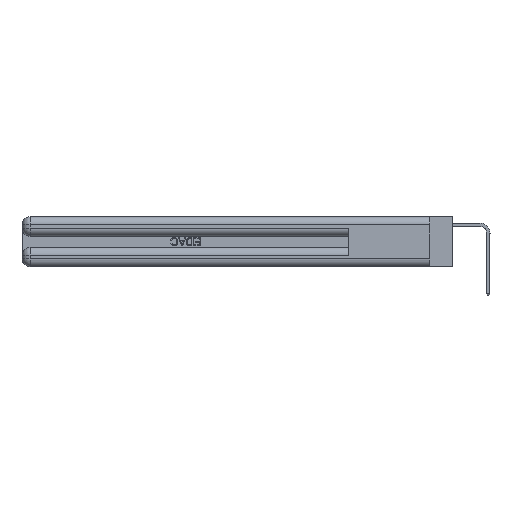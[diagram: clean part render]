
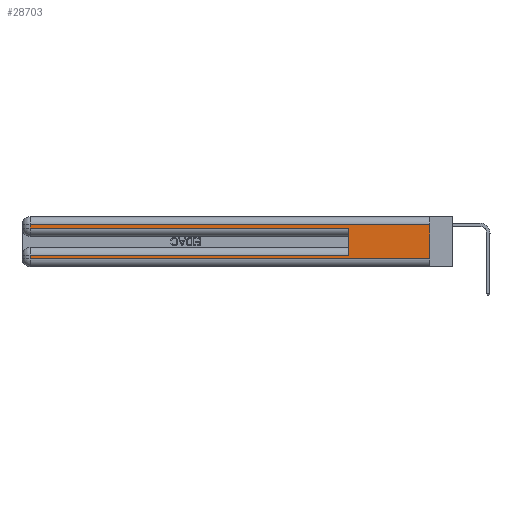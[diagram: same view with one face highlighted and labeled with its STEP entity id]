
A CAD part, left-side view. The second image highlights one B-rep face of the part: STEP entity #28703.
In plain terms, the highlighted planar face has unit normal (-1, 0, 0).
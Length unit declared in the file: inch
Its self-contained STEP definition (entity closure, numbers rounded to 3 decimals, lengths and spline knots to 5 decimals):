
#939 = CARTESIAN_POINT ( 'NONE',  ( 0., 2.94, 0.37 ) ) ;
#1863 = CARTESIAN_POINT ( 'NONE',  ( 0., 2.94, 0.285 ) ) ;
#2106 = VECTOR ( 'NONE', #22904, 39.37008 ) ;
#2240 = CARTESIAN_POINT ( 'NONE',  ( 0., 2.94, 0.31 ) ) ;
#2398 = DIRECTION ( 'NONE',  ( 0., 0., -1. ) ) ;
#3169 = VERTEX_POINT ( 'NONE', #1863 ) ;
#3526 = CARTESIAN_POINT ( 'NONE',  ( 0., 0.6, 0.085 ) ) ;
#4488 = EDGE_CURVE ( 'NONE', #3169, #23923, #26541, .T. ) ;
#4806 = VECTOR ( 'NONE', #12564, 39.37008 ) ;
#4996 = CARTESIAN_POINT ( 'NONE',  ( 0., 0., 0.06 ) ) ;
#5057 = CARTESIAN_POINT ( 'NONE',  ( 0., 0., 0.06 ) ) ;
#5118 = EDGE_CURVE ( 'NONE', #24408, #10112, #22521, .T. ) ;
#5964 = EDGE_CURVE ( 'NONE', #27807, #3169, #27616, .T. ) ;
#6028 = AXIS2_PLACEMENT_3D ( 'NONE', #30290, #17591, #2398 ) ;
#7339 = VECTOR ( 'NONE', #20966, 39.37008 ) ;
#7611 = LINE ( 'NONE', #10466, #20350 ) ;
#8115 = ORIENTED_EDGE ( 'NONE', *, *, #5118, .T. ) ;
#8141 = CARTESIAN_POINT ( 'NONE',  ( 0., 0., 0.31 ) ) ;
#9685 = VERTEX_POINT ( 'NONE', #8141 ) ;
#10076 = DIRECTION ( 'NONE',  ( 0., -1., 0. ) ) ;
#10112 = VERTEX_POINT ( 'NONE', #5057 ) ;
#10466 = CARTESIAN_POINT ( 'NONE',  ( 0., 0., 0.085 ) ) ;
#10651 = ORIENTED_EDGE ( 'NONE', *, *, #28915, .T. ) ;
#11354 = DIRECTION ( 'NONE',  ( 0., 1., 0. ) ) ;
#12394 = EDGE_LOOP ( 'NONE', ( #17187, #24290, #18702, #14174, #22247, #13338, #10651, #8115 ) ) ;
#12485 = PLANE ( 'NONE',  #6028 ) ;
#12564 = DIRECTION ( 'NONE',  ( 0., 0., -1. ) ) ;
#13027 = DIRECTION ( 'NONE',  ( 0., 1., 0. ) ) ;
#13338 = ORIENTED_EDGE ( 'NONE', *, *, #15269, .T. ) ;
#14124 = CARTESIAN_POINT ( 'NONE',  ( 0., 2.94, 0.085 ) ) ;
#14174 = ORIENTED_EDGE ( 'NONE', *, *, #4488, .T. ) ;
#15269 = EDGE_CURVE ( 'NONE', #24792, #23299, #7611, .T. ) ;
#17187 = ORIENTED_EDGE ( 'NONE', *, *, #21102, .F. ) ;
#17591 = DIRECTION ( 'NONE',  ( 1., 0., 0. ) ) ;
#18278 = LINE ( 'NONE', #27681, #4806 ) ;
#18402 = CARTESIAN_POINT ( 'NONE',  ( 0., 2.94, 0.37 ) ) ;
#18615 = LINE ( 'NONE', #939, #26958 ) ;
#18702 = ORIENTED_EDGE ( 'NONE', *, *, #5964, .T. ) ;
#20221 = CARTESIAN_POINT ( 'NONE',  ( 0., 0., 0.285 ) ) ;
#20350 = VECTOR ( 'NONE', #13027, 39.37008 ) ;
#20966 = DIRECTION ( 'NONE',  ( 0., 0., -1. ) ) ;
#21102 = EDGE_CURVE ( 'NONE', #9685, #10112, #18278, .T. ) ;
#21502 = CARTESIAN_POINT ( 'NONE',  ( 0., 0., 0.31 ) ) ;
#21755 = VECTOR ( 'NONE', #30412, 39.37008 ) ;
#22247 = ORIENTED_EDGE ( 'NONE', *, *, #25960, .F. ) ;
#22521 = LINE ( 'NONE', #4996, #21755 ) ;
#22853 = LINE ( 'NONE', #21502, #28807 ) ;
#22904 = DIRECTION ( 'NONE',  ( 0., 0., 1. ) ) ;
#23299 = VERTEX_POINT ( 'NONE', #14124 ) ;
#23923 = VERTEX_POINT ( 'NONE', #31677 ) ;
#23989 = LINE ( 'NONE', #25461, #2106 ) ;
#24212 = FACE_OUTER_BOUND ( 'NONE', #12394, .T. ) ;
#24290 = ORIENTED_EDGE ( 'NONE', *, *, #30891, .T. ) ;
#24408 = VERTEX_POINT ( 'NONE', #31744 ) ;
#24792 = VERTEX_POINT ( 'NONE', #3526 ) ;
#25461 = CARTESIAN_POINT ( 'NONE',  ( 0., 0.6, 0.145 ) ) ;
#25960 = EDGE_CURVE ( 'NONE', #24792, #23923, #23989, .T. ) ;
#26269 = DIRECTION ( 'NONE',  ( 0., 0., -1. ) ) ;
#26541 = LINE ( 'NONE', #20221, #32519 ) ;
#26958 = VECTOR ( 'NONE', #26269, 39.37008 ) ;
#27616 = LINE ( 'NONE', #18402, #7339 ) ;
#27681 = CARTESIAN_POINT ( 'NONE',  ( 0., 0., 0.37 ) ) ;
#27807 = VERTEX_POINT ( 'NONE', #2240 ) ;
#28703 = ADVANCED_FACE ( 'NONE', ( #24212 ), #12485, .F. ) ;
#28807 = VECTOR ( 'NONE', #11354, 39.37008 ) ;
#28915 = EDGE_CURVE ( 'NONE', #23299, #24408, #18615, .T. ) ;
#30290 = CARTESIAN_POINT ( 'NONE',  ( 0., 0., 0.37 ) ) ;
#30412 = DIRECTION ( 'NONE',  ( 0., -1., 0. ) ) ;
#30891 = EDGE_CURVE ( 'NONE', #9685, #27807, #22853, .T. ) ;
#31677 = CARTESIAN_POINT ( 'NONE',  ( 0., 0.6, 0.285 ) ) ;
#31744 = CARTESIAN_POINT ( 'NONE',  ( 0., 2.94, 0.06 ) ) ;
#32519 = VECTOR ( 'NONE', #10076, 39.37008 ) ;
